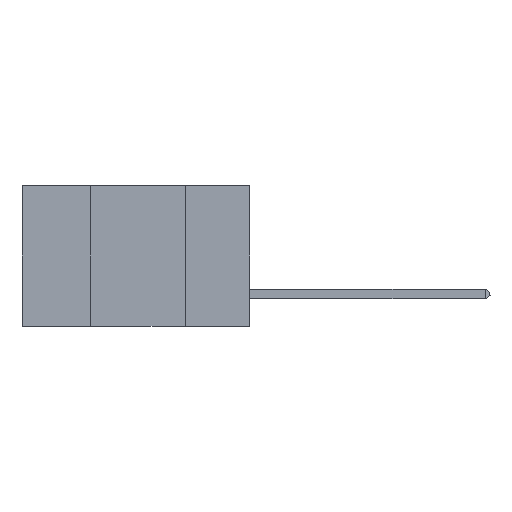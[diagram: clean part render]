
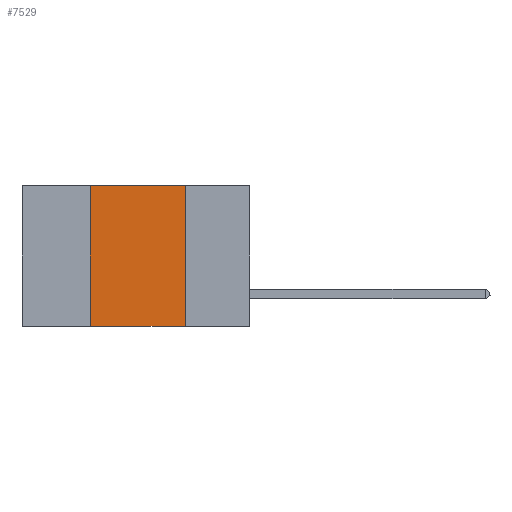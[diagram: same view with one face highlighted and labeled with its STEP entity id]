
A CAD part, left-side view. The second image highlights one B-rep face of the part: STEP entity #7529.
In plain terms, the highlighted planar face has unit normal (-1, 0, 0).
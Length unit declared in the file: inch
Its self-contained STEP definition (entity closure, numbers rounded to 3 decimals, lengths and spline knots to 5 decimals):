
#260 = DIRECTION ( 'NONE',  ( 0., 0., 1. ) ) ;
#281 = EDGE_CURVE ( 'NONE', #7247, #1506, #1451, .T. ) ;
#421 = DIRECTION ( 'NONE',  ( 0., 0., -1. ) ) ;
#531 = PLANE ( 'NONE',  #1328 ) ;
#1023 = VERTEX_POINT ( 'NONE', #2181 ) ;
#1186 = ORIENTED_EDGE ( 'NONE', *, *, #2356, .F. ) ;
#1328 = AXIS2_PLACEMENT_3D ( 'NONE', #8658, #8502, #421 ) ;
#1451 = LINE ( 'NONE', #7090, #8725 ) ;
#1506 = VERTEX_POINT ( 'NONE', #13504 ) ;
#1682 = ORIENTED_EDGE ( 'NONE', *, *, #13050, .F. ) ;
#2181 = CARTESIAN_POINT ( 'NONE',  ( 0., 0.17, 0. ) ) ;
#2356 = EDGE_CURVE ( 'NONE', #11065, #1023, #8295, .T. ) ;
#2851 = ORIENTED_EDGE ( 'NONE', *, *, #3566, .F. ) ;
#2864 = ORIENTED_EDGE ( 'NONE', *, *, #281, .T. ) ;
#3566 = EDGE_CURVE ( 'NONE', #7247, #11065, #5015, .T. ) ;
#4026 = VECTOR ( 'NONE', #9976, 39.37008 ) ;
#4731 = DIRECTION ( 'NONE',  ( 0., -1., 0. ) ) ;
#5015 = LINE ( 'NONE', #6073, #6091 ) ;
#5618 = CARTESIAN_POINT ( 'NONE',  ( 0., 0.42, -0.37 ) ) ;
#5767 = CARTESIAN_POINT ( 'NONE',  ( 0., 0.17, 0. ) ) ;
#6073 = CARTESIAN_POINT ( 'NONE',  ( 0., 0.42, 0. ) ) ;
#6091 = VECTOR ( 'NONE', #260, 39.37008 ) ;
#6916 = CARTESIAN_POINT ( 'NONE',  ( 0., 0.42, 0. ) ) ;
#7090 = CARTESIAN_POINT ( 'NONE',  ( 0., 0.6, -0.37 ) ) ;
#7247 = VERTEX_POINT ( 'NONE', #5618 ) ;
#7520 = EDGE_LOOP ( 'NONE', ( #1682, #1186, #2851, #2864 ) ) ;
#7529 = ADVANCED_FACE ( 'NONE', ( #13472 ), #531, .F. ) ;
#8295 = LINE ( 'NONE', #11805, #12613 ) ;
#8502 = DIRECTION ( 'NONE',  ( 1., 0., 0. ) ) ;
#8658 = CARTESIAN_POINT ( 'NONE',  ( 0., 0.6, 0. ) ) ;
#8725 = VECTOR ( 'NONE', #4731, 39.37008 ) ;
#9976 = DIRECTION ( 'NONE',  ( 0., 0., -1. ) ) ;
#11065 = VERTEX_POINT ( 'NONE', #6916 ) ;
#11805 = CARTESIAN_POINT ( 'NONE',  ( 0., 0.6, 0. ) ) ;
#11965 = LINE ( 'NONE', #5767, #4026 ) ;
#12613 = VECTOR ( 'NONE', #14180, 39.37008 ) ;
#13050 = EDGE_CURVE ( 'NONE', #1023, #1506, #11965, .T. ) ;
#13472 = FACE_OUTER_BOUND ( 'NONE', #7520, .T. ) ;
#13504 = CARTESIAN_POINT ( 'NONE',  ( 0., 0.17, -0.37 ) ) ;
#14180 = DIRECTION ( 'NONE',  ( 0., -1., 0. ) ) ;
